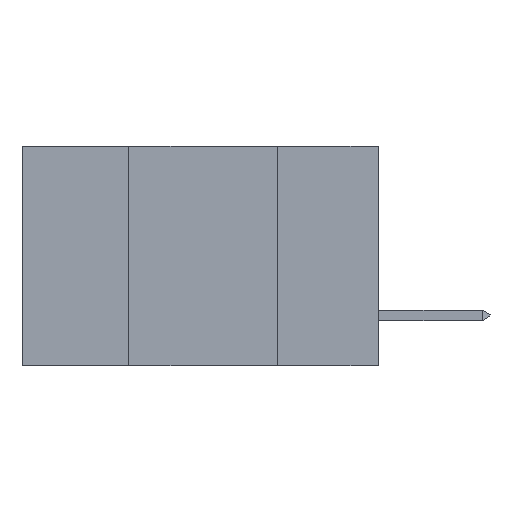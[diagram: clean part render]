
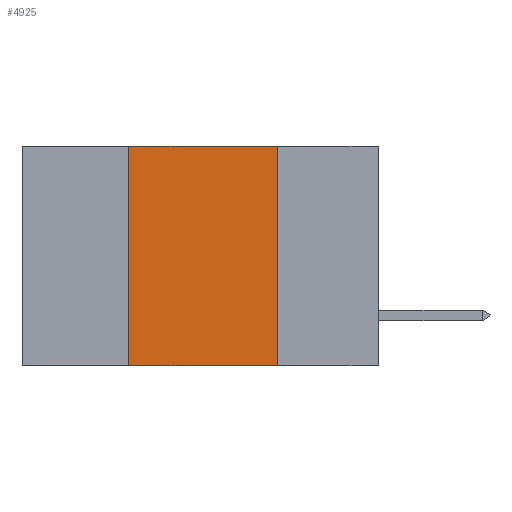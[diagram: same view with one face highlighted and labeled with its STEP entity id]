
A CAD part, left-side view. The second image highlights one B-rep face of the part: STEP entity #4925.
In plain terms, the highlighted planar face has unit normal (-1, 0, 0).
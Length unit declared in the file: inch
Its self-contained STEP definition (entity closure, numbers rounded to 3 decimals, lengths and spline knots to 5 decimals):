
#1244 = VERTEX_POINT ( 'NONE', #13112 ) ;
#1351 = DIRECTION ( 'NONE',  ( 0., 0., -1. ) ) ;
#1743 = VECTOR ( 'NONE', #11377, 39.37008 ) ;
#2606 = LINE ( 'NONE', #18620, #19018 ) ;
#2899 = CARTESIAN_POINT ( 'NONE',  ( 0., 0.17, 0. ) ) ;
#2986 = LINE ( 'NONE', #8831, #16677 ) ;
#4515 = DIRECTION ( 'NONE',  ( 0., 0., -1. ) ) ;
#4525 = VERTEX_POINT ( 'NONE', #21047 ) ;
#4925 = ADVANCED_FACE ( 'NONE', ( #5255 ), #9253, .F. ) ;
#5255 = FACE_OUTER_BOUND ( 'NONE', #15854, .T. ) ;
#5618 = DIRECTION ( 'NONE',  ( 1., 0., 0. ) ) ;
#6299 = ORIENTED_EDGE ( 'NONE', *, *, #17108, .F. ) ;
#7887 = ORIENTED_EDGE ( 'NONE', *, *, #14572, .F. ) ;
#8489 = EDGE_CURVE ( 'NONE', #4525, #24237, #10208, .T. ) ;
#8831 = CARTESIAN_POINT ( 'NONE',  ( 0., 0.6, -0.37 ) ) ;
#9253 = PLANE ( 'NONE',  #25297 ) ;
#9565 = CARTESIAN_POINT ( 'NONE',  ( 0., 0.42, 0. ) ) ;
#10208 = LINE ( 'NONE', #11266, #15983 ) ;
#10434 = ORIENTED_EDGE ( 'NONE', *, *, #14429, .T. ) ;
#11266 = CARTESIAN_POINT ( 'NONE',  ( 0., 0.6, 0. ) ) ;
#11377 = DIRECTION ( 'NONE',  ( 0., 0., 1. ) ) ;
#11489 = CARTESIAN_POINT ( 'NONE',  ( 0., 0.6, 0. ) ) ;
#12748 = LINE ( 'NONE', #9565, #1743 ) ;
#13112 = CARTESIAN_POINT ( 'NONE',  ( 0., 0.17, -0.37 ) ) ;
#13148 = DIRECTION ( 'NONE',  ( 0., -1., 0. ) ) ;
#14429 = EDGE_CURVE ( 'NONE', #23127, #1244, #2986, .T. ) ;
#14572 = EDGE_CURVE ( 'NONE', #23127, #4525, #12748, .T. ) ;
#15854 = EDGE_LOOP ( 'NONE', ( #6299, #15864, #7887, #10434 ) ) ;
#15864 = ORIENTED_EDGE ( 'NONE', *, *, #8489, .F. ) ;
#15983 = VECTOR ( 'NONE', #13148, 39.37008 ) ;
#16677 = VECTOR ( 'NONE', #22635, 39.37008 ) ;
#17108 = EDGE_CURVE ( 'NONE', #24237, #1244, #2606, .T. ) ;
#18620 = CARTESIAN_POINT ( 'NONE',  ( 0., 0.17, 0. ) ) ;
#19018 = VECTOR ( 'NONE', #4515, 39.37008 ) ;
#21047 = CARTESIAN_POINT ( 'NONE',  ( 0., 0.42, 0. ) ) ;
#21597 = CARTESIAN_POINT ( 'NONE',  ( 0., 0.42, -0.37 ) ) ;
#22635 = DIRECTION ( 'NONE',  ( 0., -1., 0. ) ) ;
#23127 = VERTEX_POINT ( 'NONE', #21597 ) ;
#24237 = VERTEX_POINT ( 'NONE', #2899 ) ;
#25297 = AXIS2_PLACEMENT_3D ( 'NONE', #11489, #5618, #1351 ) ;
